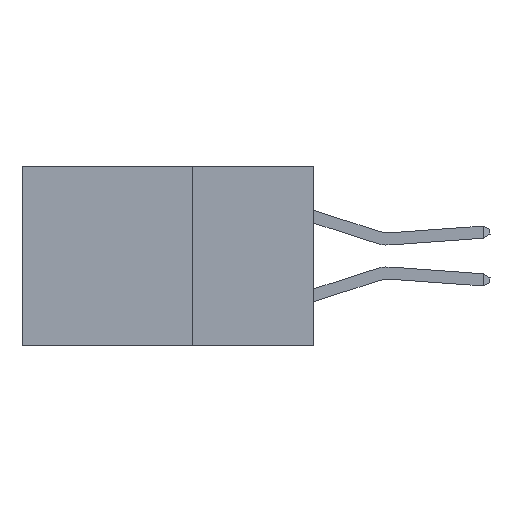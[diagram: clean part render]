
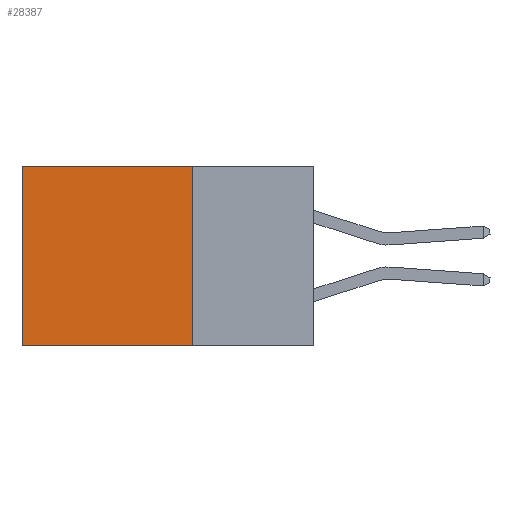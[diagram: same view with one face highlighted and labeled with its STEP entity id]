
A CAD part, left-side view. The second image highlights one B-rep face of the part: STEP entity #28387.
In plain terms, the highlighted planar face has unit normal (-1, 0, 0).
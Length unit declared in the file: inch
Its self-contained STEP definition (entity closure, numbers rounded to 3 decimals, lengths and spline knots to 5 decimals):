
#981 = DIRECTION ( 'NONE',  ( 1., 0., 0. ) ) ;
#1718 = EDGE_CURVE ( 'NONE', #11963, #25767, #29625, .T. ) ;
#2085 = CARTESIAN_POINT ( 'NONE',  ( 0.2875, 0.6, -0.37 ) ) ;
#3380 = CARTESIAN_POINT ( 'NONE',  ( 0.2875, 0.25, 0. ) ) ;
#3573 = CARTESIAN_POINT ( 'NONE',  ( 0.2875, 0.25, 0. ) ) ;
#3598 = VECTOR ( 'NONE', #28519, 39.37008 ) ;
#3760 = VECTOR ( 'NONE', #27909, 39.37008 ) ;
#5083 = ORIENTED_EDGE ( 'NONE', *, *, #1718, .T. ) ;
#8355 = DIRECTION ( 'NONE',  ( 0., 0., -1. ) ) ;
#9014 = VECTOR ( 'NONE', #21406, 39.37008 ) ;
#9191 = CARTESIAN_POINT ( 'NONE',  ( 0.2875, 0.25, 0. ) ) ;
#9776 = LINE ( 'NONE', #9191, #9014 ) ;
#11273 = EDGE_CURVE ( 'NONE', #24819, #18511, #9776, .T. ) ;
#11963 = VERTEX_POINT ( 'NONE', #12497 ) ;
#12497 = CARTESIAN_POINT ( 'NONE',  ( 0.2875, 0.6, 0. ) ) ;
#16938 = LINE ( 'NONE', #21723, #27294 ) ;
#16995 = FACE_OUTER_BOUND ( 'NONE', #20427, .T. ) ;
#17426 = ORIENTED_EDGE ( 'NONE', *, *, #11273, .F. ) ;
#17526 = LINE ( 'NONE', #3380, #3760 ) ;
#18511 = VERTEX_POINT ( 'NONE', #25986 ) ;
#18800 = CARTESIAN_POINT ( 'NONE',  ( 0.2875, 0.25, 0. ) ) ;
#18802 = ORIENTED_EDGE ( 'NONE', *, *, #19897, .T. ) ;
#19897 = EDGE_CURVE ( 'NONE', #24819, #11963, #17526, .T. ) ;
#19963 = AXIS2_PLACEMENT_3D ( 'NONE', #3573, #981, #8355 ) ;
#20427 = EDGE_LOOP ( 'NONE', ( #5083, #23684, #17426, #18802 ) ) ;
#21406 = DIRECTION ( 'NONE',  ( 0., 0., -1. ) ) ;
#21723 = CARTESIAN_POINT ( 'NONE',  ( 0.2875, 0.25, -0.37 ) ) ;
#23075 = PLANE ( 'NONE',  #19963 ) ;
#23684 = ORIENTED_EDGE ( 'NONE', *, *, #29405, .F. ) ;
#24819 = VERTEX_POINT ( 'NONE', #18800 ) ;
#25767 = VERTEX_POINT ( 'NONE', #2085 ) ;
#25986 = CARTESIAN_POINT ( 'NONE',  ( 0.2875, 0.25, -0.37 ) ) ;
#26208 = CARTESIAN_POINT ( 'NONE',  ( 0.2875, 0.6, 0. ) ) ;
#27294 = VECTOR ( 'NONE', #29016, 39.37008 ) ;
#27909 = DIRECTION ( 'NONE',  ( 0., 1., 0. ) ) ;
#28387 = ADVANCED_FACE ( 'NONE', ( #16995 ), #23075, .F. ) ;
#28519 = DIRECTION ( 'NONE',  ( 0., 0., -1. ) ) ;
#29016 = DIRECTION ( 'NONE',  ( 0., 1., 0. ) ) ;
#29405 = EDGE_CURVE ( 'NONE', #18511, #25767, #16938, .T. ) ;
#29625 = LINE ( 'NONE', #26208, #3598 ) ;
